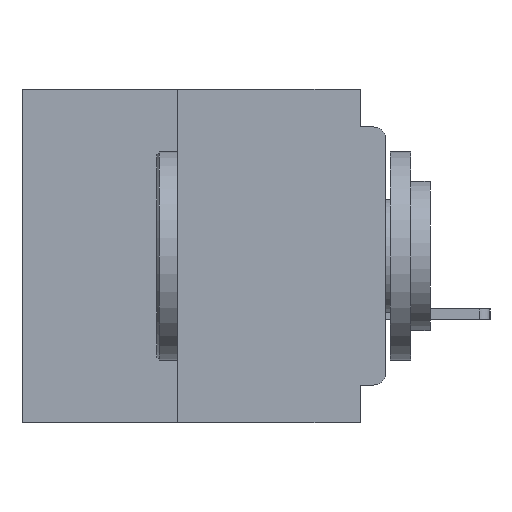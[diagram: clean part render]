
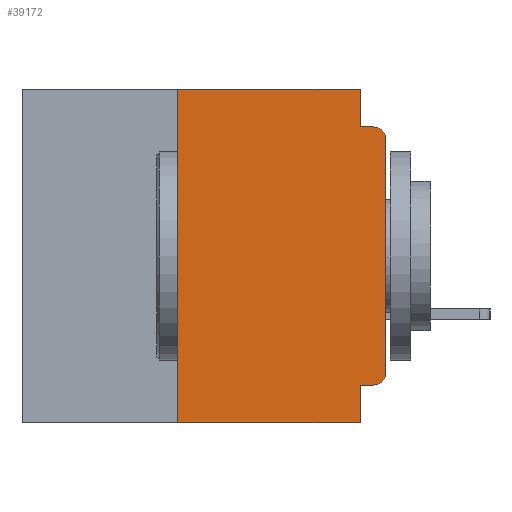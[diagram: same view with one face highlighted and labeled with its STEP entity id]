
A CAD part, left-side view. The second image highlights one B-rep face of the part: STEP entity #39172.
In plain terms, the highlighted planar face has unit normal (-1, 0, 0).
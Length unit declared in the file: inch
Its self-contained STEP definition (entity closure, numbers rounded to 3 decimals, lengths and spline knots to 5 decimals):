
#1302 = LINE ( 'NONE', #25191, #25898 ) ;
#1618 = VECTOR ( 'NONE', #16649, 39.37008 ) ;
#2656 = EDGE_CURVE ( 'NONE', #51516, #46043, #50819, .T. ) ;
#2951 = CARTESIAN_POINT ( 'NONE',  ( 0., 0.031, -0.4 ) ) ;
#9600 = EDGE_CURVE ( 'NONE', #34920, #51516, #42366, .T. ) ;
#11735 = VERTEX_POINT ( 'NONE', #29091 ) ;
#12424 = LINE ( 'NONE', #27273, #62431 ) ;
#12949 = DIRECTION ( 'NONE',  ( 0., 0., -1. ) ) ;
#13349 = VECTOR ( 'NONE', #15161, 39.37008 ) ;
#15161 = DIRECTION ( 'NONE',  ( 0., 1., 0. ) ) ;
#16649 = DIRECTION ( 'NONE',  ( 0., 0., -1. ) ) ;
#17855 = AXIS2_PLACEMENT_3D ( 'NONE', #50392, #21446, #55256 ) ;
#18913 = DIRECTION ( 'NONE',  ( 0., -1., 0. ) ) ;
#19597 = CARTESIAN_POINT ( 'NONE',  ( 0., 0.25, 0. ) ) ;
#19619 = VECTOR ( 'NONE', #51658, 39.37008 ) ;
#20907 = EDGE_CURVE ( 'NONE', #11735, #32687, #54913, .T. ) ;
#21102 = CARTESIAN_POINT ( 'NONE',  ( 0., 0.015, -0.06 ) ) ;
#21193 = VERTEX_POINT ( 'NONE', #28485 ) ;
#21446 = DIRECTION ( 'NONE',  ( -1., 0., 0. ) ) ;
#21557 = ORIENTED_EDGE ( 'NONE', *, *, #44991, .F. ) ;
#22395 = EDGE_CURVE ( 'NONE', #34920, #40129, #39168, .T. ) ;
#22966 = ORIENTED_EDGE ( 'NONE', *, *, #25214, .T. ) ;
#24283 = EDGE_CURVE ( 'NONE', #28509, #11735, #41168, .T. ) ;
#24419 = AXIS2_PLACEMENT_3D ( 'NONE', #21102, #54898, #25986 ) ;
#25191 = CARTESIAN_POINT ( 'NONE',  ( 0., 0., -0.045 ) ) ;
#25214 = EDGE_CURVE ( 'NONE', #46043, #21193, #62170, .T. ) ;
#25898 = VECTOR ( 'NONE', #44605, 39.37008 ) ;
#25986 = DIRECTION ( 'NONE',  ( 0., 0., -1. ) ) ;
#27273 = CARTESIAN_POINT ( 'NONE',  ( 0., 0.25, -0.4 ) ) ;
#27719 = AXIS2_PLACEMENT_3D ( 'NONE', #56332, #41999, #12949 ) ;
#28485 = CARTESIAN_POINT ( 'NONE',  ( 0., 0.015, -0.045 ) ) ;
#28509 = VERTEX_POINT ( 'NONE', #19597 ) ;
#29012 = VECTOR ( 'NONE', #30744, 39.37008 ) ;
#29091 = CARTESIAN_POINT ( 'NONE',  ( 0., 0.031, 0. ) ) ;
#29700 = DIRECTION ( 'NONE',  ( 0., 0., 1. ) ) ;
#29980 = EDGE_CURVE ( 'NONE', #49943, #61003, #30522, .T. ) ;
#30189 = CARTESIAN_POINT ( 'NONE',  ( 0., 0., 0. ) ) ;
#30494 = EDGE_CURVE ( 'NONE', #32687, #21193, #1302, .T. ) ;
#30522 = LINE ( 'NONE', #40448, #29012 ) ;
#30744 = DIRECTION ( 'NONE',  ( 0., -1., 0. ) ) ;
#30868 = CARTESIAN_POINT ( 'NONE',  ( 0., 0.015, -0.355 ) ) ;
#30892 = CARTESIAN_POINT ( 'NONE',  ( 0., 0.031, -0.045 ) ) ;
#32500 = LINE ( 'NONE', #2951, #19619 ) ;
#32687 = VERTEX_POINT ( 'NONE', #30892 ) ;
#34487 = CARTESIAN_POINT ( 'NONE',  ( 0., 0., -0.355 ) ) ;
#34920 = VERTEX_POINT ( 'NONE', #30868 ) ;
#35001 = VECTOR ( 'NONE', #29700, 39.37008 ) ;
#36953 = ORIENTED_EDGE ( 'NONE', *, *, #22395, .F. ) ;
#39168 = LINE ( 'NONE', #34487, #13349 ) ;
#39172 = ADVANCED_FACE ( 'NONE', ( #55207 ), #61186, .F. ) ;
#40129 = VERTEX_POINT ( 'NONE', #46598 ) ;
#40448 = CARTESIAN_POINT ( 'NONE',  ( 0., 0.437, -0.4 ) ) ;
#41168 = LINE ( 'NONE', #47843, #53981 ) ;
#41999 = DIRECTION ( 'NONE',  ( 1., 0., 0. ) ) ;
#42366 = CIRCLE ( 'NONE', #17855, 0.015 ) ;
#42561 = CARTESIAN_POINT ( 'NONE',  ( 0., 0., -0.34 ) ) ;
#44605 = DIRECTION ( 'NONE',  ( 0., -1., 0. ) ) ;
#44991 = EDGE_CURVE ( 'NONE', #49943, #28509, #12424, .T. ) ;
#45898 = ORIENTED_EDGE ( 'NONE', *, *, #20907, .F. ) ;
#46043 = VERTEX_POINT ( 'NONE', #53962 ) ;
#46598 = CARTESIAN_POINT ( 'NONE',  ( 0., 0.031, -0.355 ) ) ;
#47843 = CARTESIAN_POINT ( 'NONE',  ( 0., 0.437, 0. ) ) ;
#48455 = ORIENTED_EDGE ( 'NONE', *, *, #2656, .T. ) ;
#48738 = EDGE_CURVE ( 'NONE', #40129, #61003, #32500, .T. ) ;
#49943 = VERTEX_POINT ( 'NONE', #60998 ) ;
#50392 = CARTESIAN_POINT ( 'NONE',  ( 0., 0.015, -0.34 ) ) ;
#50436 = CARTESIAN_POINT ( 'NONE',  ( 0., 0.031, 0. ) ) ;
#50819 = LINE ( 'NONE', #30189, #35001 ) ;
#51165 = ORIENTED_EDGE ( 'NONE', *, *, #9600, .T. ) ;
#51516 = VERTEX_POINT ( 'NONE', #42561 ) ;
#51658 = DIRECTION ( 'NONE',  ( 0., 0., -1. ) ) ;
#51832 = ORIENTED_EDGE ( 'NONE', *, *, #48738, .F. ) ;
#52453 = ORIENTED_EDGE ( 'NONE', *, *, #24283, .F. ) ;
#53407 = ORIENTED_EDGE ( 'NONE', *, *, #30494, .F. ) ;
#53962 = CARTESIAN_POINT ( 'NONE',  ( 0., 0., -0.06 ) ) ;
#53981 = VECTOR ( 'NONE', #18913, 39.37008 ) ;
#54825 = ORIENTED_EDGE ( 'NONE', *, *, #29980, .T. ) ;
#54898 = DIRECTION ( 'NONE',  ( -1., 0., 0. ) ) ;
#54913 = LINE ( 'NONE', #50436, #1618 ) ;
#55207 = FACE_OUTER_BOUND ( 'NONE', #59370, .T. ) ;
#55256 = DIRECTION ( 'NONE',  ( 0., 0., -1. ) ) ;
#56332 = CARTESIAN_POINT ( 'NONE',  ( 0., 0.437, 0. ) ) ;
#56414 = CARTESIAN_POINT ( 'NONE',  ( 0., 0.031, -0.4 ) ) ;
#59370 = EDGE_LOOP ( 'NONE', ( #48455, #22966, #53407, #45898, #52453, #21557, #54825, #51832, #36953, #51165 ) ) ;
#60998 = CARTESIAN_POINT ( 'NONE',  ( 0., 0.25, -0.4 ) ) ;
#61003 = VERTEX_POINT ( 'NONE', #56414 ) ;
#61029 = DIRECTION ( 'NONE',  ( 0., 0., 1. ) ) ;
#61186 = PLANE ( 'NONE',  #27719 ) ;
#62170 = CIRCLE ( 'NONE', #24419, 0.015 ) ;
#62431 = VECTOR ( 'NONE', #61029, 39.37008 ) ;
